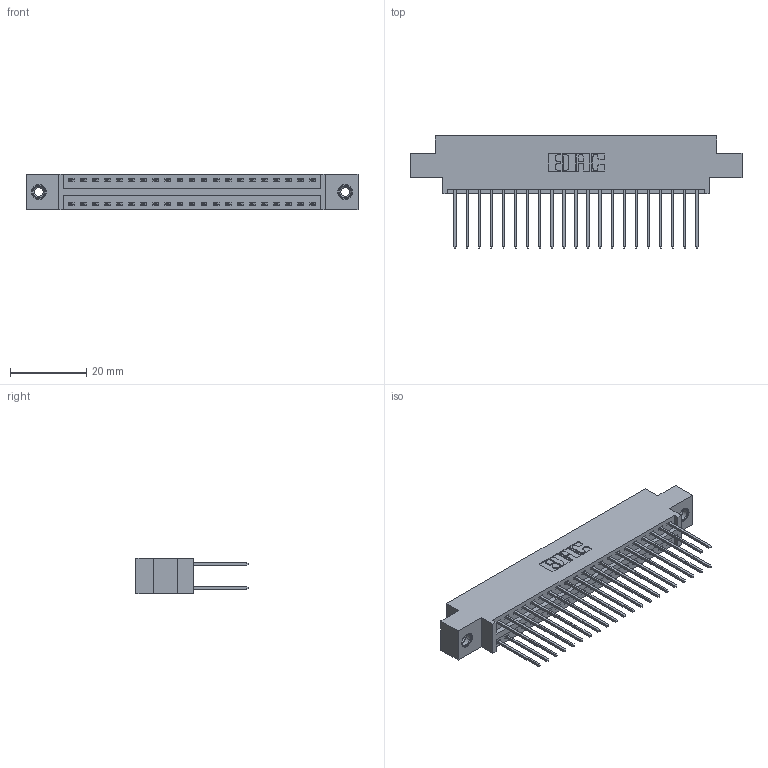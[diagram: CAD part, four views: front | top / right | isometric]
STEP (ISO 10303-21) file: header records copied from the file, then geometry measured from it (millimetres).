
FILE_DESCRIPTION (( 'STEP AP203' ), '1' );
FILE_NAME ('346-042-540-808.STEP', '2022-05-20T04:35:08', ( '' ), ( '' ), 'SwSTEP 2.0', 'SolidWorks 2020', '' );
FILE_SCHEMA (( 'CONFIG_CONTROL_DESIGN' ));
Length unit declared in the file: inch
Products named in the file (4): 346 Part_0.170 Offset - 0.156 Dia-TI; 346-042-540-808; 345-292-001_345-293-140; 345-250-001_345-250-003-102
Assembly tree (45 placements, depth 2):
  346-042-540-808
    346 Part_0.170 Offset - 0.156 Dia-TI
    345-292-001_345-293-140  x42
    345-250-001_345-250-003-102  x2
Bounding box: 87.25 x 29.46 x 9.4 mm (x, y, z)
Volume: 8342.9 mm3; surface area: 12090.5 mm2
Topology: 45 solids, 45 shells, 2370 faces, 6987 edges, 4594 vertices
Faces by surface type: plane 1582, cylinder 772, cone 12, torus 4
Entity records: 17868 total; most frequent: CARTESIAN_POINT 2959, ORIENTED_EDGE 2886, DIRECTION 2685, EDGE_CURVE 1443, VECTOR 1207, LINE 1207, VERTEX_POINT 956, AXIS2_PLACEMENT_3D 739
